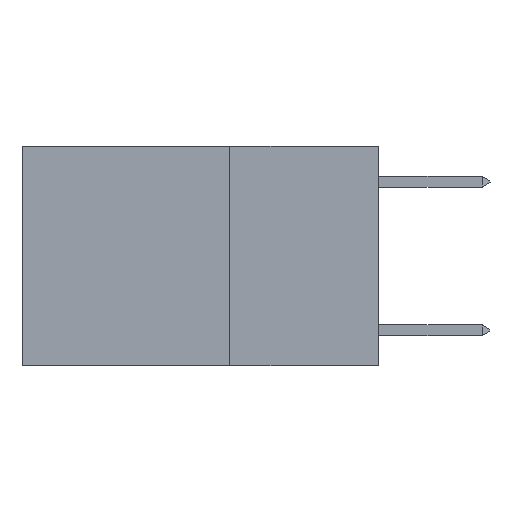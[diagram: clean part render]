
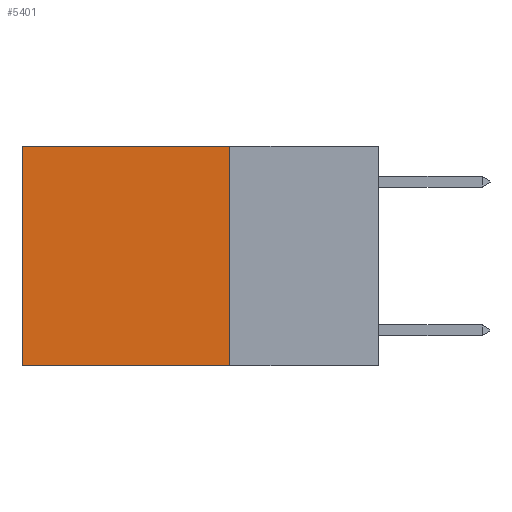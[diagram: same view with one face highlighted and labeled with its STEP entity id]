
A CAD part, left-side view. The second image highlights one B-rep face of the part: STEP entity #5401.
In plain terms, the highlighted planar face has unit normal (-1, 0, 0).
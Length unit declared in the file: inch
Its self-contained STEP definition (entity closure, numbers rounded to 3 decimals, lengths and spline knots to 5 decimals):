
#18 = VECTOR ( 'NONE', #663, 39.37008 ) ;
#108 = LINE ( 'NONE', #665, #18 ) ;
#132 = DIRECTION ( 'NONE',  ( 1., 0., 0. ) ) ;
#138 = VECTOR ( 'NONE', #7627, 39.37008 ) ;
#215 = PLANE ( 'NONE',  #277 ) ;
#250 = CARTESIAN_POINT ( 'NONE',  ( 0.2625, 0.25, 0. ) ) ;
#259 = LINE ( 'NONE', #9336, #6414 ) ;
#277 = AXIS2_PLACEMENT_3D ( 'NONE', #250, #132, #6624 ) ;
#300 = LINE ( 'NONE', #2943, #138 ) ;
#663 = DIRECTION ( 'NONE',  ( 0., 0., -1. ) ) ;
#665 = CARTESIAN_POINT ( 'NONE',  ( 0.2625, 0.6, 0. ) ) ;
#827 = FACE_OUTER_BOUND ( 'NONE', #8247, .T. ) ;
#1070 = LINE ( 'NONE', #4769, #5645 ) ;
#1220 = CARTESIAN_POINT ( 'NONE',  ( 0.2625, 0.6, -0.37 ) ) ;
#1500 = CARTESIAN_POINT ( 'NONE',  ( 0.2625, 0.25, -0.37 ) ) ;
#1544 = CARTESIAN_POINT ( 'NONE',  ( 0.2625, 0.25, 0. ) ) ;
#1657 = VERTEX_POINT ( 'NONE', #1500 ) ;
#1698 = EDGE_CURVE ( 'NONE', #3895, #4760, #108, .T. ) ;
#2943 = CARTESIAN_POINT ( 'NONE',  ( 0.2625, 0.25, 0. ) ) ;
#3152 = EDGE_CURVE ( 'NONE', #7500, #1657, #300, .T. ) ;
#3862 = ORIENTED_EDGE ( 'NONE', *, *, #1698, .T. ) ;
#3895 = VERTEX_POINT ( 'NONE', #7976 ) ;
#4760 = VERTEX_POINT ( 'NONE', #1220 ) ;
#4769 = CARTESIAN_POINT ( 'NONE',  ( 0.2625, 0.25, -0.37 ) ) ;
#4814 = DIRECTION ( 'NONE',  ( 0., 1., 0. ) ) ;
#5401 = ADVANCED_FACE ( 'NONE', ( #827 ), #215, .F. ) ;
#5492 = EDGE_CURVE ( 'NONE', #7500, #3895, #259, .T. ) ;
#5645 = VECTOR ( 'NONE', #4814, 39.37008 ) ;
#5860 = ORIENTED_EDGE ( 'NONE', *, *, #6398, .F. ) ;
#6398 = EDGE_CURVE ( 'NONE', #1657, #4760, #1070, .T. ) ;
#6414 = VECTOR ( 'NONE', #9382, 39.37008 ) ;
#6624 = DIRECTION ( 'NONE',  ( 0., 0., -1. ) ) ;
#7118 = ORIENTED_EDGE ( 'NONE', *, *, #5492, .T. ) ;
#7500 = VERTEX_POINT ( 'NONE', #1544 ) ;
#7627 = DIRECTION ( 'NONE',  ( 0., 0., -1. ) ) ;
#7976 = CARTESIAN_POINT ( 'NONE',  ( 0.2625, 0.6, 0. ) ) ;
#8207 = ORIENTED_EDGE ( 'NONE', *, *, #3152, .F. ) ;
#8247 = EDGE_LOOP ( 'NONE', ( #3862, #5860, #8207, #7118 ) ) ;
#9336 = CARTESIAN_POINT ( 'NONE',  ( 0.2625, 0.25, 0. ) ) ;
#9382 = DIRECTION ( 'NONE',  ( 0., 1., 0. ) ) ;
